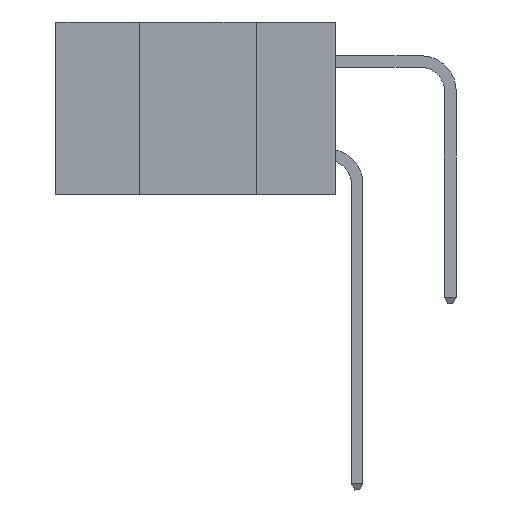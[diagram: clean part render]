
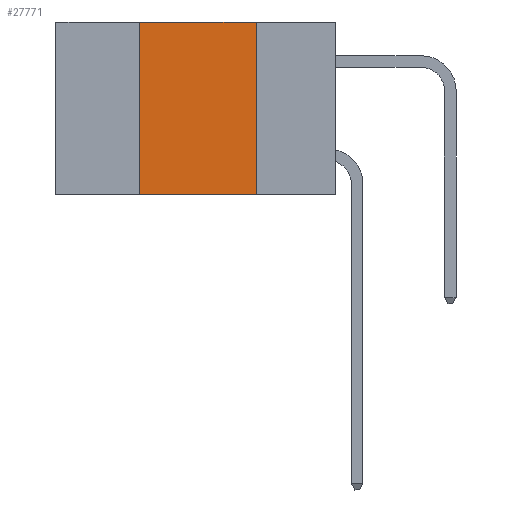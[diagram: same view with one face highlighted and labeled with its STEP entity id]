
A CAD part, left-side view. The second image highlights one B-rep face of the part: STEP entity #27771.
In plain terms, the highlighted planar face has unit normal (-1, 0, 0).
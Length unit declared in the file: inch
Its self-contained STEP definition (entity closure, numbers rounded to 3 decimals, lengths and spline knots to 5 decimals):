
#2009 = FACE_OUTER_BOUND ( 'NONE', #12354, .T. ) ;
#4614 = ORIENTED_EDGE ( 'NONE', *, *, #14008, .F. ) ;
#5325 = CARTESIAN_POINT ( 'NONE',  ( 0., 0.17, 0. ) ) ;
#5447 = PLANE ( 'NONE',  #31262 ) ;
#5566 = DIRECTION ( 'NONE',  ( 0., 0., -1. ) ) ;
#7551 = EDGE_CURVE ( 'NONE', #15532, #18629, #34008, .T. ) ;
#7887 = VERTEX_POINT ( 'NONE', #12219 ) ;
#7914 = LINE ( 'NONE', #31691, #29487 ) ;
#8190 = CARTESIAN_POINT ( 'NONE',  ( 0., 0.6, -0.37 ) ) ;
#8373 = VERTEX_POINT ( 'NONE', #25335 ) ;
#10181 = EDGE_CURVE ( 'NONE', #7887, #18629, #10593, .T. ) ;
#10593 = LINE ( 'NONE', #8190, #30365 ) ;
#12219 = CARTESIAN_POINT ( 'NONE',  ( 0., 0.42, -0.37 ) ) ;
#12354 = EDGE_LOOP ( 'NONE', ( #25381, #4614, #19694, #21433 ) ) ;
#13008 = CARTESIAN_POINT ( 'NONE',  ( 0., 0.17, -0.37 ) ) ;
#14008 = EDGE_CURVE ( 'NONE', #8373, #15532, #25038, .T. ) ;
#14852 = DIRECTION ( 'NONE',  ( 0., 0., 1. ) ) ;
#15532 = VERTEX_POINT ( 'NONE', #5325 ) ;
#18629 = VERTEX_POINT ( 'NONE', #13008 ) ;
#19161 = CARTESIAN_POINT ( 'NONE',  ( 0., 0.17, 0. ) ) ;
#19614 = EDGE_CURVE ( 'NONE', #7887, #8373, #7914, .T. ) ;
#19682 = CARTESIAN_POINT ( 'NONE',  ( 0., 0.6, 0. ) ) ;
#19694 = ORIENTED_EDGE ( 'NONE', *, *, #19614, .F. ) ;
#21433 = ORIENTED_EDGE ( 'NONE', *, *, #10181, .T. ) ;
#21601 = DIRECTION ( 'NONE',  ( 0., -1., 0. ) ) ;
#21946 = DIRECTION ( 'NONE',  ( 0., 0., -1. ) ) ;
#22341 = DIRECTION ( 'NONE',  ( 0., -1., 0. ) ) ;
#22478 = DIRECTION ( 'NONE',  ( 1., 0., 0. ) ) ;
#24145 = VECTOR ( 'NONE', #21601, 39.37008 ) ;
#25038 = LINE ( 'NONE', #32784, #24145 ) ;
#25335 = CARTESIAN_POINT ( 'NONE',  ( 0., 0.42, 0. ) ) ;
#25381 = ORIENTED_EDGE ( 'NONE', *, *, #7551, .F. ) ;
#26564 = VECTOR ( 'NONE', #21946, 39.37008 ) ;
#27771 = ADVANCED_FACE ( 'NONE', ( #2009 ), #5447, .F. ) ;
#29487 = VECTOR ( 'NONE', #14852, 39.37008 ) ;
#30365 = VECTOR ( 'NONE', #22341, 39.37008 ) ;
#31262 = AXIS2_PLACEMENT_3D ( 'NONE', #19682, #22478, #5566 ) ;
#31691 = CARTESIAN_POINT ( 'NONE',  ( 0., 0.42, 0. ) ) ;
#32784 = CARTESIAN_POINT ( 'NONE',  ( 0., 0.6, 0. ) ) ;
#34008 = LINE ( 'NONE', #19161, #26564 ) ;
